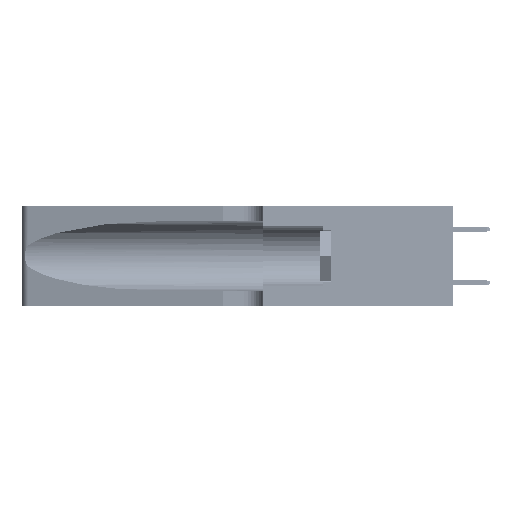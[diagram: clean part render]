
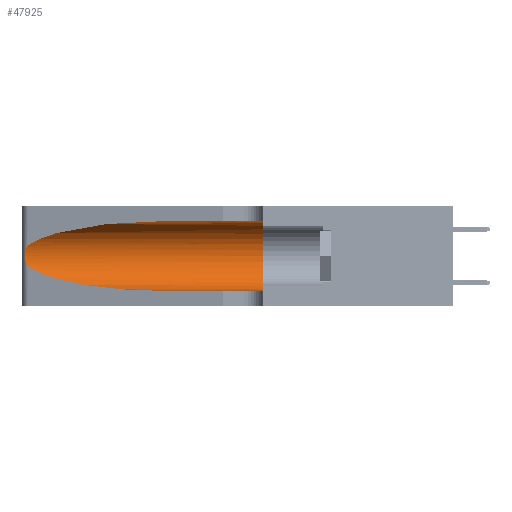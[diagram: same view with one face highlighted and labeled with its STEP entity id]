
A CAD part, left-side view. The second image highlights one B-rep face of the part: STEP entity #47925.
In plain terms, the highlighted cylindrical face has radius 3.308 mm (diameter 6.617 mm), a partial arc.
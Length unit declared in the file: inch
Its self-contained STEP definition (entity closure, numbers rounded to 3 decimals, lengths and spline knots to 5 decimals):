
#404 = LINE ( 'NONE', #21259, #16606 ) ;
#1352 =( BOUNDED_CURVE ( )  B_SPLINE_CURVE ( 3, ( #51426, #25237, #31051, #51685 ),
 .UNSPECIFIED., .F., .F. ) 
 B_SPLINE_CURVE_WITH_KNOTS ( ( 4, 4 ),
 ( 1.5708, 2.84003 ),
 .UNSPECIFIED. ) 
 CURVE ( )  GEOMETRIC_REPRESENTATION_ITEM ( )  RATIONAL_B_SPLINE_CURVE ( ( 1., 0.87, 0.87, 1. ) ) 
 REPRESENTATION_ITEM ( '' )  );
#2172 = CYLINDRICAL_SURFACE ( 'NONE', #24994, 0.13025 ) ;
#3024 = VERTEX_POINT ( 'NONE', #13903 ) ;
#3180 = CARTESIAN_POINT ( 'NONE',  ( 0.1305, 0.72297, 0.05475 ) ) ;
#4426 = DIRECTION ( 'NONE',  ( 0., 1., 0. ) ) ;
#5268 = EDGE_LOOP ( 'NONE', ( #34208, #24806, #52014, #37790, #49462, #17409 ) ) ;
#5908 = CARTESIAN_POINT ( 'NONE',  ( 0.25639, 1.23184, 0.21858 ) ) ;
#6092 = EDGE_CURVE ( 'NONE', #36782, #3024, #52693, .T. ) ;
#6998 = CARTESIAN_POINT ( 'NONE',  ( 0.25555, 1.22993, 0.14849 ) ) ;
#7261 = CARTESIAN_POINT ( 'NONE',  ( 0.26017, 1.23833, 0.17102 ) ) ;
#10201 = CARTESIAN_POINT ( 'NONE',  ( 0.1305, 1.61858, 0.185 ) ) ;
#10245 = EDGE_CURVE ( 'NONE', #38599, #48000, #43405, .T. ) ;
#10729 = FACE_OUTER_BOUND ( 'NONE', #5268, .T. ) ;
#11286 = CARTESIAN_POINT ( 'NONE',  ( 0.25639, 1.23186, 0.15144 ) ) ;
#11539 = CARTESIAN_POINT ( 'NONE',  ( 0.25856, 1.23593, 0.16098 ) ) ;
#12714 = DIRECTION ( 'NONE',  ( 0., 0., 1. ) ) ;
#12816 = VERTEX_POINT ( 'NONE', #13993 ) ;
#13433 = CARTESIAN_POINT ( 'NONE',  ( 0.25787, 1.23484, 0.2124 ) ) ;
#13903 = CARTESIAN_POINT ( 'NONE',  ( 0.1305, 0.35, 0.05475 ) ) ;
#13993 = CARTESIAN_POINT ( 'NONE',  ( 0.25487, 1.22718, 0.22369 ) ) ;
#14771 = DIRECTION ( 'NONE',  ( 0., 0., -1. ) ) ;
#16606 = VECTOR ( 'NONE', #33070, 39.37008 ) ;
#17409 = ORIENTED_EDGE ( 'NONE', *, *, #34206, .F. ) ;
#17763 = EDGE_CURVE ( 'NONE', #40503, #12816, #1352, .T. ) ;
#18960 = CARTESIAN_POINT ( 'NONE',  ( 0.2373, 1.15595, 0.08982 ) ) ;
#19300 = CARTESIAN_POINT ( 'NONE',  ( 0.26075, 1.23896, 0.178 ) ) ;
#20632 = EDGE_CURVE ( 'NONE', #48000, #3024, #20653, .T. ) ;
#20653 = LINE ( 'NONE', #36978, #51153 ) ;
#21259 = CARTESIAN_POINT ( 'NONE',  ( 0.1305, 1.61858, 0.31525 ) ) ;
#21343 = B_SPLINE_CURVE_WITH_KNOTS ( 'NONE', 3,
 ( #46594, #42567, #5908, #13433, #46067, #35906, #52264, #19300, #7261, #11539, #48237, #11286, #6998, #27062 ),
 .UNSPECIFIED., .F., .F.,
 ( 4, 2, 2, 2, 2, 2, 4 ),
 ( 0., 0.00027, 0.00053, 0.00107, 0.0016, 0.00187, 0.00214 ),
 .UNSPECIFIED. ) ;
#23587 = DIRECTION ( 'NONE',  ( 0., -1., 0. ) ) ;
#23788 = CARTESIAN_POINT ( 'NONE',  ( 0.18966, 0.96281, 0.05475 ) ) ;
#23944 = CARTESIAN_POINT ( 'NONE',  ( 0.1305, 0.35, 0.31525 ) ) ;
#24806 = ORIENTED_EDGE ( 'NONE', *, *, #34397, .T. ) ;
#24994 = AXIS2_PLACEMENT_3D ( 'NONE', #10201, #23587, #14771 ) ;
#25237 = CARTESIAN_POINT ( 'NONE',  ( 0.18966, 0.96281, 0.31525 ) ) ;
#27062 = CARTESIAN_POINT ( 'NONE',  ( 0.25487, 1.22718, 0.14631 ) ) ;
#30934 = CARTESIAN_POINT ( 'NONE',  ( 0.1305, 0.72297, 0.31525 ) ) ;
#31051 = CARTESIAN_POINT ( 'NONE',  ( 0.2373, 1.15595, 0.28018 ) ) ;
#33070 = DIRECTION ( 'NONE',  ( 0., -1., 0. ) ) ;
#34206 = EDGE_CURVE ( 'NONE', #40503, #36782, #404, .T. ) ;
#34208 = ORIENTED_EDGE ( 'NONE', *, *, #17763, .T. ) ;
#34397 = EDGE_CURVE ( 'NONE', #12816, #38599, #21343, .T. ) ;
#35906 = CARTESIAN_POINT ( 'NONE',  ( 0.26018, 1.23835, 0.19895 ) ) ;
#36782 = VERTEX_POINT ( 'NONE', #23944 ) ;
#36978 = CARTESIAN_POINT ( 'NONE',  ( 0.1305, 1.61858, 0.05475 ) ) ;
#37790 = ORIENTED_EDGE ( 'NONE', *, *, #20632, .T. ) ;
#38507 = CARTESIAN_POINT ( 'NONE',  ( 0.25487, 1.22718, 0.14631 ) ) ;
#38599 = VERTEX_POINT ( 'NONE', #51276 ) ;
#40503 = VERTEX_POINT ( 'NONE', #30934 ) ;
#41498 = AXIS2_PLACEMENT_3D ( 'NONE', #52660, #4426, #12714 ) ;
#42567 = CARTESIAN_POINT ( 'NONE',  ( 0.25555, 1.22994, 0.2215 ) ) ;
#43405 =( BOUNDED_CURVE ( )  B_SPLINE_CURVE ( 3, ( #38507, #18960, #23788, #3180 ),
 .UNSPECIFIED., .F., .F. ) 
 B_SPLINE_CURVE_WITH_KNOTS ( ( 4, 4 ),
 ( 3.44316, 4.71239 ),
 .UNSPECIFIED. ) 
 CURVE ( )  GEOMETRIC_REPRESENTATION_ITEM ( )  RATIONAL_B_SPLINE_CURVE ( ( 1., 0.87, 0.87, 1. ) ) 
 REPRESENTATION_ITEM ( '' )  );
#46067 = CARTESIAN_POINT ( 'NONE',  ( 0.25854, 1.2359, 0.20912 ) ) ;
#46594 = CARTESIAN_POINT ( 'NONE',  ( 0.25487, 1.22718, 0.22369 ) ) ;
#47702 = CARTESIAN_POINT ( 'NONE',  ( 0.1305, 0.72297, 0.05475 ) ) ;
#47925 = ADVANCED_FACE ( 'NONE', ( #10729 ), #2172, .F. ) ;
#48000 = VERTEX_POINT ( 'NONE', #47702 ) ;
#48237 = CARTESIAN_POINT ( 'NONE',  ( 0.25789, 1.23486, 0.15765 ) ) ;
#48792 = DIRECTION ( 'NONE',  ( 0., -1., 0. ) ) ;
#49462 = ORIENTED_EDGE ( 'NONE', *, *, #6092, .F. ) ;
#51153 = VECTOR ( 'NONE', #48792, 39.37008 ) ;
#51276 = CARTESIAN_POINT ( 'NONE',  ( 0.25487, 1.22718, 0.14631 ) ) ;
#51426 = CARTESIAN_POINT ( 'NONE',  ( 0.1305, 0.72297, 0.31525 ) ) ;
#51685 = CARTESIAN_POINT ( 'NONE',  ( 0.25487, 1.22718, 0.22369 ) ) ;
#52014 = ORIENTED_EDGE ( 'NONE', *, *, #10245, .T. ) ;
#52264 = CARTESIAN_POINT ( 'NONE',  ( 0.26075, 1.23896, 0.19203 ) ) ;
#52660 = CARTESIAN_POINT ( 'NONE',  ( 0.1305, 0.35, 0.185 ) ) ;
#52693 = CIRCLE ( 'NONE', #41498, 0.13025 ) ;
